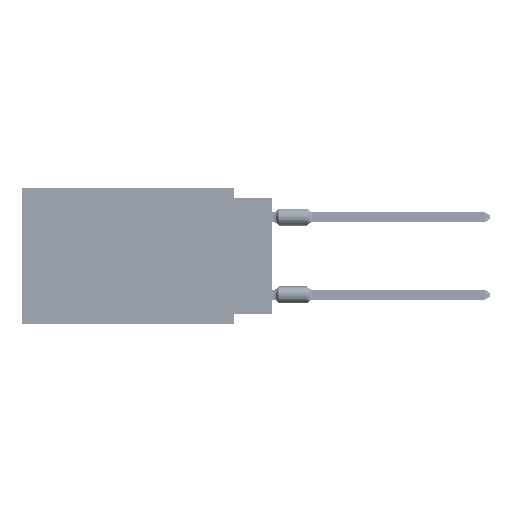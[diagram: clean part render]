
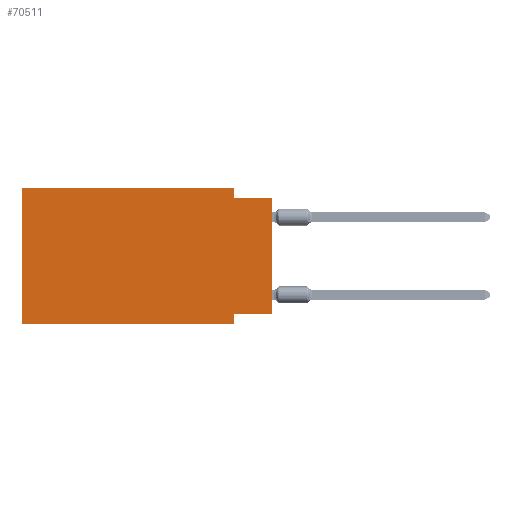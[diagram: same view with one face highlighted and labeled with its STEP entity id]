
A CAD part, left-side view. The second image highlights one B-rep face of the part: STEP entity #70511.
In plain terms, the highlighted planar face has unit normal (-1, 0, 0).
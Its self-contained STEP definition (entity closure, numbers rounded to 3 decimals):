
#4134 = CARTESIAN_POINT ( 'NONE',  ( 0., 0., -8.255 ) ) ;
#4899 = DIRECTION ( 'NONE',  ( 0., -1., 0. ) ) ;
#5579 = VECTOR ( 'NONE', #75354, 1000. ) ;
#6620 = EDGE_CURVE ( 'NONE', #31735, #81803, #30371, .T. ) ;
#7063 = CARTESIAN_POINT ( 'NONE',  ( 0., 2.54, -8.89 ) ) ;
#8314 = ORIENTED_EDGE ( 'NONE', *, *, #6620, .F. ) ;
#10017 = LINE ( 'NONE', #48972, #80562 ) ;
#12168 = VERTEX_POINT ( 'NONE', #4134 ) ;
#12605 = PLANE ( 'NONE',  #35722 ) ;
#15596 = DIRECTION ( 'NONE',  ( 0., -1., 0. ) ) ;
#17717 = CARTESIAN_POINT ( 'NONE',  ( 0., 16.383, -8.89 ) ) ;
#18599 = FACE_OUTER_BOUND ( 'NONE', #42655, .T. ) ;
#18743 = VERTEX_POINT ( 'NONE', #64658 ) ;
#21448 = VERTEX_POINT ( 'NONE', #7063 ) ;
#23648 = EDGE_CURVE ( 'NONE', #82630, #21448, #10017, .T. ) ;
#23884 = VERTEX_POINT ( 'NONE', #52735 ) ;
#24197 = DIRECTION ( 'NONE',  ( 0., 0., -1. ) ) ;
#24784 = ORIENTED_EDGE ( 'NONE', *, *, #33880, .T. ) ;
#27331 = CARTESIAN_POINT ( 'NONE',  ( 0., 16.383, 0. ) ) ;
#28462 = LINE ( 'NONE', #73859, #46015 ) ;
#28874 = DIRECTION ( 'NONE',  ( 0., 1., 0. ) ) ;
#29834 = DIRECTION ( 'NONE',  ( 0., -1., 0. ) ) ;
#30371 = LINE ( 'NONE', #50488, #5579 ) ;
#31735 = VERTEX_POINT ( 'NONE', #74111 ) ;
#32562 = VERTEX_POINT ( 'NONE', #68227 ) ;
#33880 = EDGE_CURVE ( 'NONE', #31735, #21448, #70374, .T. ) ;
#34432 = ORIENTED_EDGE ( 'NONE', *, *, #65119, .F. ) ;
#35434 = ORIENTED_EDGE ( 'NONE', *, *, #63490, .F. ) ;
#35722 = AXIS2_PLACEMENT_3D ( 'NONE', #82849, #83267, #24197 ) ;
#37905 = LINE ( 'NONE', #64008, #66321 ) ;
#39988 = EDGE_CURVE ( 'NONE', #12168, #32562, #41570, .T. ) ;
#41570 = LINE ( 'NONE', #54841, #74116 ) ;
#42655 = EDGE_LOOP ( 'NONE', ( #58119, #34432, #35434, #66061, #8314, #24784, #73547, #63883 ) ) ;
#43709 = EDGE_CURVE ( 'NONE', #12168, #82630, #28462, .T. ) ;
#44661 = VECTOR ( 'NONE', #4899, 1000. ) ;
#46015 = VECTOR ( 'NONE', #28874, 1000. ) ;
#48129 = LINE ( 'NONE', #74253, #51637 ) ;
#48972 = CARTESIAN_POINT ( 'NONE',  ( 0., 2.54, -8.89 ) ) ;
#50488 = CARTESIAN_POINT ( 'NONE',  ( 0., 16.383, 0. ) ) ;
#51637 = VECTOR ( 'NONE', #15596, 1000. ) ;
#52735 = CARTESIAN_POINT ( 'NONE',  ( 0., 2.54, -0.635 ) ) ;
#53131 = CARTESIAN_POINT ( 'NONE',  ( 0., 2.54, -8.255 ) ) ;
#54841 = CARTESIAN_POINT ( 'NONE',  ( 0., 0., 0. ) ) ;
#55520 = CARTESIAN_POINT ( 'NONE',  ( 0., 16.383, 0. ) ) ;
#56223 = DIRECTION ( 'NONE',  ( 0., 0., -1. ) ) ;
#58119 = ORIENTED_EDGE ( 'NONE', *, *, #39988, .T. ) ;
#63490 = EDGE_CURVE ( 'NONE', #18743, #23884, #37905, .T. ) ;
#63589 = DIRECTION ( 'NONE',  ( 0., 0., -1. ) ) ;
#63883 = ORIENTED_EDGE ( 'NONE', *, *, #43709, .F. ) ;
#64008 = CARTESIAN_POINT ( 'NONE',  ( 0., 2.54, 0. ) ) ;
#64658 = CARTESIAN_POINT ( 'NONE',  ( 0., 2.54, 0. ) ) ;
#65119 = EDGE_CURVE ( 'NONE', #23884, #32562, #48129, .T. ) ;
#66061 = ORIENTED_EDGE ( 'NONE', *, *, #66348, .F. ) ;
#66321 = VECTOR ( 'NONE', #63589, 1000. ) ;
#66348 = EDGE_CURVE ( 'NONE', #81803, #18743, #76065, .T. ) ;
#68227 = CARTESIAN_POINT ( 'NONE',  ( 0., 0., -0.635 ) ) ;
#68260 = VECTOR ( 'NONE', #29834, 1000. ) ;
#70374 = LINE ( 'NONE', #17717, #44661 ) ;
#70511 = ADVANCED_FACE ( 'NONE', ( #18599 ), #12605, .F. ) ;
#73547 = ORIENTED_EDGE ( 'NONE', *, *, #23648, .F. ) ;
#73859 = CARTESIAN_POINT ( 'NONE',  ( 0., 0., -8.255 ) ) ;
#74111 = CARTESIAN_POINT ( 'NONE',  ( 0., 16.383, -8.89 ) ) ;
#74116 = VECTOR ( 'NONE', #80952, 1000. ) ;
#74253 = CARTESIAN_POINT ( 'NONE',  ( 0., 0., -0.635 ) ) ;
#75354 = DIRECTION ( 'NONE',  ( 0., 0., 1. ) ) ;
#76065 = LINE ( 'NONE', #55520, #68260 ) ;
#80562 = VECTOR ( 'NONE', #56223, 1000. ) ;
#80952 = DIRECTION ( 'NONE',  ( 0., 0., 1. ) ) ;
#81803 = VERTEX_POINT ( 'NONE', #27331 ) ;
#82630 = VERTEX_POINT ( 'NONE', #53131 ) ;
#82849 = CARTESIAN_POINT ( 'NONE',  ( 0., 16.383, 0. ) ) ;
#83267 = DIRECTION ( 'NONE',  ( 1., 0., 0. ) ) ;
